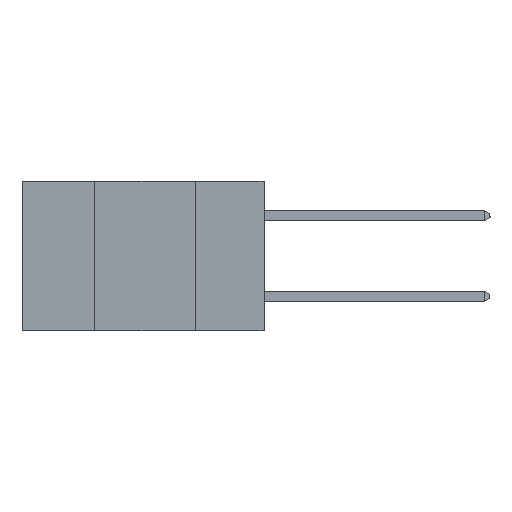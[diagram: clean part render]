
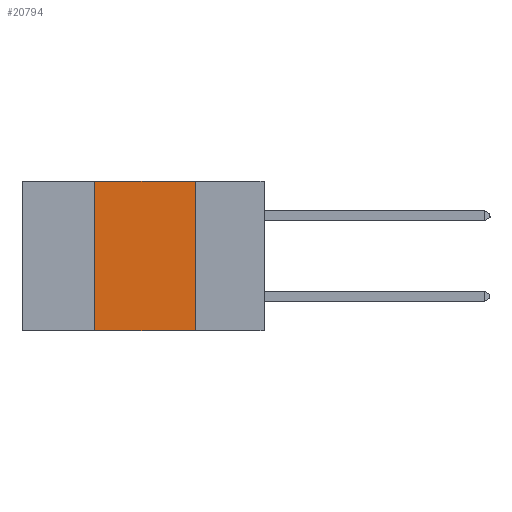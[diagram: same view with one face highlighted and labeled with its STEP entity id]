
A CAD part, left-side view. The second image highlights one B-rep face of the part: STEP entity #20794.
In plain terms, the highlighted planar face has unit normal (-1, 0, 0).
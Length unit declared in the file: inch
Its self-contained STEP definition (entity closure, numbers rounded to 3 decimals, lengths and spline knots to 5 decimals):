
#142 = EDGE_CURVE ( 'NONE', #21254, #8933, #8355, .T. ) ;
#414 = CARTESIAN_POINT ( 'NONE',  ( 0., 0.17, 0. ) ) ;
#1492 = PLANE ( 'NONE',  #19979 ) ;
#1858 = LINE ( 'NONE', #5760, #6927 ) ;
#2485 = EDGE_CURVE ( 'NONE', #12511, #21254, #1858, .T. ) ;
#2669 = CARTESIAN_POINT ( 'NONE',  ( 0., 0.6, -0.37 ) ) ;
#2674 = VECTOR ( 'NONE', #18805, 39.37008 ) ;
#3128 = CARTESIAN_POINT ( 'NONE',  ( 0., 0.17, -0.37 ) ) ;
#4084 = CARTESIAN_POINT ( 'NONE',  ( 0., 0.42, -0.37 ) ) ;
#4802 = DIRECTION ( 'NONE',  ( 0., 0., 1. ) ) ;
#5760 = CARTESIAN_POINT ( 'NONE',  ( 0., 0.42, 0. ) ) ;
#5837 = DIRECTION ( 'NONE',  ( 1., 0., 0. ) ) ;
#6927 = VECTOR ( 'NONE', #4802, 39.37008 ) ;
#7621 = ORIENTED_EDGE ( 'NONE', *, *, #142, .F. ) ;
#8058 = EDGE_LOOP ( 'NONE', ( #23410, #7621, #8258, #19996 ) ) ;
#8258 = ORIENTED_EDGE ( 'NONE', *, *, #2485, .F. ) ;
#8355 = LINE ( 'NONE', #19295, #2674 ) ;
#8933 = VERTEX_POINT ( 'NONE', #16850 ) ;
#9969 = VERTEX_POINT ( 'NONE', #3128 ) ;
#12511 = VERTEX_POINT ( 'NONE', #4084 ) ;
#12721 = LINE ( 'NONE', #414, #17617 ) ;
#13890 = EDGE_CURVE ( 'NONE', #8933, #9969, #12721, .T. ) ;
#16339 = CARTESIAN_POINT ( 'NONE',  ( 0., 0.6, 0. ) ) ;
#16850 = CARTESIAN_POINT ( 'NONE',  ( 0., 0.17, 0. ) ) ;
#16974 = DIRECTION ( 'NONE',  ( 0., -1., 0. ) ) ;
#17372 = DIRECTION ( 'NONE',  ( 0., 0., -1. ) ) ;
#17617 = VECTOR ( 'NONE', #17372, 39.37008 ) ;
#18805 = DIRECTION ( 'NONE',  ( 0., -1., 0. ) ) ;
#19295 = CARTESIAN_POINT ( 'NONE',  ( 0., 0.6, 0. ) ) ;
#19979 = AXIS2_PLACEMENT_3D ( 'NONE', #16339, #5837, #20441 ) ;
#19996 = ORIENTED_EDGE ( 'NONE', *, *, #23928, .T. ) ;
#20299 = VECTOR ( 'NONE', #16974, 39.37008 ) ;
#20441 = DIRECTION ( 'NONE',  ( 0., 0., -1. ) ) ;
#20794 = ADVANCED_FACE ( 'NONE', ( #26847 ), #1492, .F. ) ;
#21254 = VERTEX_POINT ( 'NONE', #21773 ) ;
#21773 = CARTESIAN_POINT ( 'NONE',  ( 0., 0.42, 0. ) ) ;
#23410 = ORIENTED_EDGE ( 'NONE', *, *, #13890, .F. ) ;
#23928 = EDGE_CURVE ( 'NONE', #12511, #9969, #26259, .T. ) ;
#26259 = LINE ( 'NONE', #2669, #20299 ) ;
#26847 = FACE_OUTER_BOUND ( 'NONE', #8058, .T. ) ;
